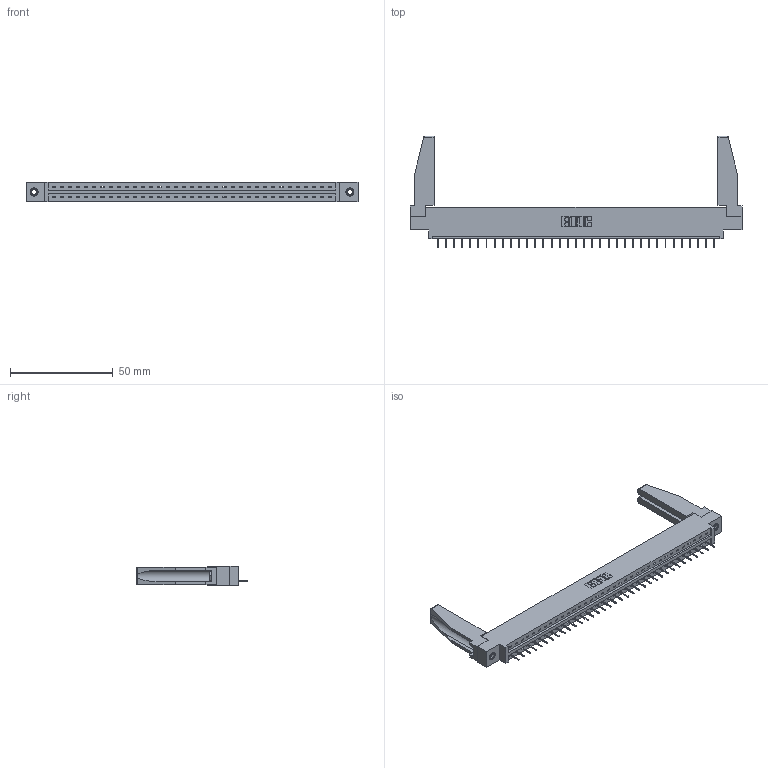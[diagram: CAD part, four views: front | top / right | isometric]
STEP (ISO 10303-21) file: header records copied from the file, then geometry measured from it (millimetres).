
FILE_DESCRIPTION (( 'STEP AP203' ), '1' );
FILE_NAME ('337-035-524-678.STEP', '2019-10-01T12:54:32', ( '' ), ( '' ), 'SwSTEP 2.0', 'SolidWorks 2016', '' );
FILE_SCHEMA (( 'CONFIG_CONTROL_DESIGN' ));
Length unit declared in the file: inch
Products named in the file (5): 345-250-001_345-250-001-102; 337-035-524-678; 345-292-001_345-293-124; 337 Part_0.170 Offset - 0.156 Dia-TI; 307-220-078
Assembly tree (40 placements, depth 2):
  337-035-524-678
    337 Part_0.170 Offset - 0.156 Dia-TI
    345-292-001_345-293-124  x35
    345-250-001_345-250-001-102  x2
    307-220-078  x2
Bounding box: 161.7 x 54.49 x 9.4 mm (x, y, z)
Volume: 20455.6 mm3; surface area: 20419.6 mm2
Topology: 40 solids, 40 shells, 2558 faces, 7373 edges, 4766 vertices
Faces by surface type: plane 1978, cylinder 564, cone 12, torus 4
Entity records: 29568 total; most frequent: CARTESIAN_POINT 5141, ORIENTED_EDGE 5068, DIRECTION 4352, EDGE_CURVE 2534, LINE 2372, VECTOR 2372, VERTEX_POINT 1680, AXIS2_PLACEMENT_3D 990
